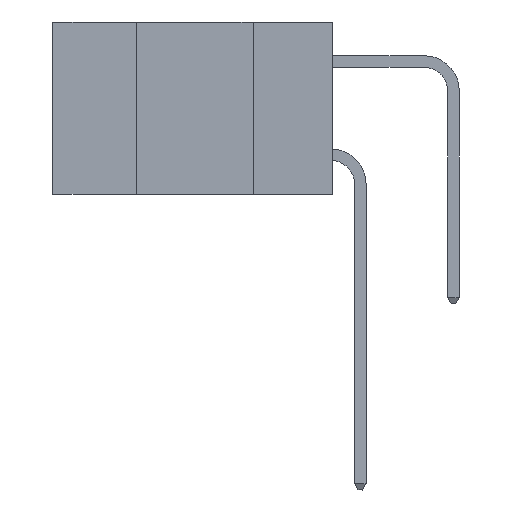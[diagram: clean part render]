
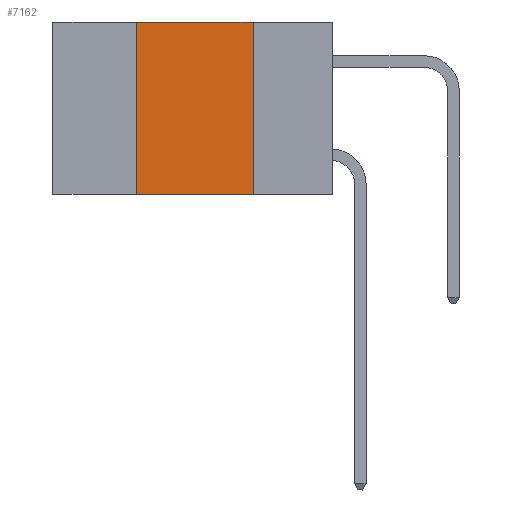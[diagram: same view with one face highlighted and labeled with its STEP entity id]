
A CAD part, left-side view. The second image highlights one B-rep face of the part: STEP entity #7162.
In plain terms, the highlighted planar face has unit normal (-1, 0, 0).
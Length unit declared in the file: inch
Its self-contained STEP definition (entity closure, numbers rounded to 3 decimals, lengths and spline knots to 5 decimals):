
#238 = VERTEX_POINT ( 'NONE', #12180 ) ;
#248 = DIRECTION ( 'NONE',  ( 1., 0., 0. ) ) ;
#1396 = DIRECTION ( 'NONE',  ( 0., 0., -1. ) ) ;
#1437 = EDGE_CURVE ( 'NONE', #12863, #5901, #7027, .T. ) ;
#2706 = PLANE ( 'NONE',  #10066 ) ;
#2935 = VECTOR ( 'NONE', #9826, 39.37008 ) ;
#4041 = FACE_OUTER_BOUND ( 'NONE', #7468, .T. ) ;
#4043 = CARTESIAN_POINT ( 'NONE',  ( 0., 0.42, 0. ) ) ;
#4939 = ORIENTED_EDGE ( 'NONE', *, *, #1437, .F. ) ;
#5113 = DIRECTION ( 'NONE',  ( 0., 0., -1. ) ) ;
#5546 = CARTESIAN_POINT ( 'NONE',  ( 0., 0.17, -0.37 ) ) ;
#5760 = VECTOR ( 'NONE', #9366, 39.37008 ) ;
#5901 = VERTEX_POINT ( 'NONE', #4043 ) ;
#6086 = DIRECTION ( 'NONE',  ( 0., 0., 1. ) ) ;
#6204 = VERTEX_POINT ( 'NONE', #5546 ) ;
#7027 = LINE ( 'NONE', #8416, #9303 ) ;
#7162 = ADVANCED_FACE ( 'NONE', ( #4041 ), #2706, .F. ) ;
#7468 = EDGE_LOOP ( 'NONE', ( #13984, #8801, #4939, #13058 ) ) ;
#7949 = CARTESIAN_POINT ( 'NONE',  ( 0., 0.42, -0.37 ) ) ;
#8416 = CARTESIAN_POINT ( 'NONE',  ( 0., 0.42, 0. ) ) ;
#8598 = LINE ( 'NONE', #10526, #5760 ) ;
#8801 = ORIENTED_EDGE ( 'NONE', *, *, #12913, .F. ) ;
#9303 = VECTOR ( 'NONE', #6086, 39.37008 ) ;
#9366 = DIRECTION ( 'NONE',  ( 0., -1., 0. ) ) ;
#9826 = DIRECTION ( 'NONE',  ( 0., -1., 0. ) ) ;
#10066 = AXIS2_PLACEMENT_3D ( 'NONE', #12305, #248, #5113 ) ;
#10526 = CARTESIAN_POINT ( 'NONE',  ( 0., 0.6, 0. ) ) ;
#10843 = LINE ( 'NONE', #11206, #2935 ) ;
#11033 = LINE ( 'NONE', #13410, #14285 ) ;
#11206 = CARTESIAN_POINT ( 'NONE',  ( 0., 0.6, -0.37 ) ) ;
#12180 = CARTESIAN_POINT ( 'NONE',  ( 0., 0.17, 0. ) ) ;
#12305 = CARTESIAN_POINT ( 'NONE',  ( 0., 0.6, 0. ) ) ;
#12863 = VERTEX_POINT ( 'NONE', #7949 ) ;
#12913 = EDGE_CURVE ( 'NONE', #5901, #238, #8598, .T. ) ;
#13058 = ORIENTED_EDGE ( 'NONE', *, *, #13230, .T. ) ;
#13230 = EDGE_CURVE ( 'NONE', #12863, #6204, #10843, .T. ) ;
#13410 = CARTESIAN_POINT ( 'NONE',  ( 0., 0.17, 0. ) ) ;
#13494 = EDGE_CURVE ( 'NONE', #238, #6204, #11033, .T. ) ;
#13984 = ORIENTED_EDGE ( 'NONE', *, *, #13494, .F. ) ;
#14285 = VECTOR ( 'NONE', #1396, 39.37008 ) ;
